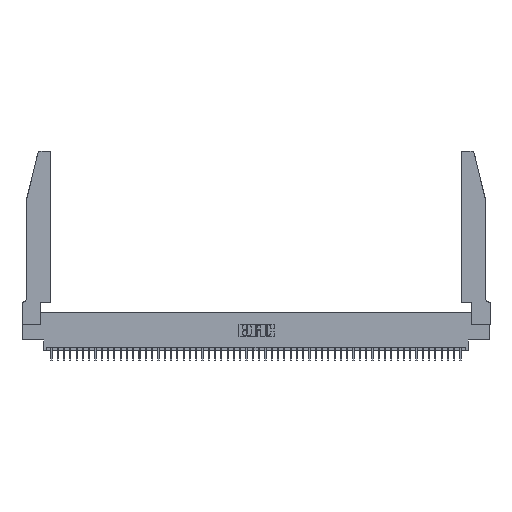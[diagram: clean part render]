
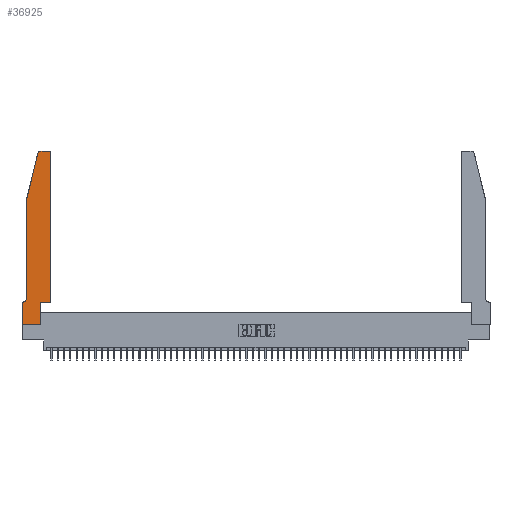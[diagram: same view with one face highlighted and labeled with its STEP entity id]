
A CAD part, top view. The second image highlights one B-rep face of the part: STEP entity #36925.
In plain terms, the highlighted planar face has unit normal (0, 0, 1).
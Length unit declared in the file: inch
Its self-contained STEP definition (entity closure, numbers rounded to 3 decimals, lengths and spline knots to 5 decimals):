
#589 = DIRECTION ( 'NONE',  ( -1., 0., 0. ) ) ;
#664 = CARTESIAN_POINT ( 'NONE',  ( 0.4505, 2.72, 0.37 ) ) ;
#1329 = VERTEX_POINT ( 'NONE', #664 ) ;
#1554 = VERTEX_POINT ( 'NONE', #31294 ) ;
#1745 = EDGE_CURVE ( 'NONE', #17024, #6309, #14048, .T. ) ;
#1891 = EDGE_CURVE ( 'NONE', #22762, #1329, #19160, .T. ) ;
#2009 = ORIENTED_EDGE ( 'NONE', *, *, #38502, .T. ) ;
#2164 = EDGE_CURVE ( 'NONE', #41203, #17024, #21786, .T. ) ;
#2355 = VERTEX_POINT ( 'NONE', #8171 ) ;
#2985 = CARTESIAN_POINT ( 'NONE',  ( 0., 0.35, 0.37 ) ) ;
#3336 = VERTEX_POINT ( 'NONE', #47160 ) ;
#3424 = EDGE_CURVE ( 'NONE', #1329, #51830, #41658, .T. ) ;
#3543 = VECTOR ( 'NONE', #29038, 39.37008 ) ;
#3907 = DIRECTION ( 'NONE',  ( 0., 0., 1. ) ) ;
#4087 = DIRECTION ( 'NONE',  ( 0., 1., 0. ) ) ;
#4681 = ORIENTED_EDGE ( 'NONE', *, *, #37167, .T. ) ;
#5021 = DIRECTION ( 'NONE',  ( 0., 0., -1. ) ) ;
#5131 = ORIENTED_EDGE ( 'NONE', *, *, #1891, .T. ) ;
#6309 = VERTEX_POINT ( 'NONE', #47322 ) ;
#6726 = DIRECTION ( 'NONE',  ( 1., 0., 0. ) ) ;
#6755 = FACE_OUTER_BOUND ( 'NONE', #8197, .T. ) ;
#8171 = CARTESIAN_POINT ( 'NONE',  ( 0.0055, 0.35, 0.37 ) ) ;
#8197 = EDGE_LOOP ( 'NONE', ( #2009, #19649, #50811, #50943, #4681, #10469, #21205, #13644, #23918, #22284, #5131, #49922 ) ) ;
#9561 = EDGE_CURVE ( 'NONE', #21285, #1554, #14188, .T. ) ;
#10469 = ORIENTED_EDGE ( 'NONE', *, *, #12463, .T. ) ;
#10592 = DIRECTION ( 'NONE',  ( -0.239, -0.971, 0. ) ) ;
#12463 = EDGE_CURVE ( 'NONE', #2355, #21559, #24625, .T. ) ;
#12718 = VECTOR ( 'NONE', #13935, 39.37008 ) ;
#12909 = VECTOR ( 'NONE', #47338, 39.37008 ) ;
#13644 = ORIENTED_EDGE ( 'NONE', *, *, #41360, .T. ) ;
#13935 = DIRECTION ( 'NONE',  ( 0., -1., 0. ) ) ;
#14048 = LINE ( 'NONE', #34669, #45701 ) ;
#14188 = LINE ( 'NONE', #51188, #12909 ) ;
#15741 = CARTESIAN_POINT ( 'NONE',  ( 0.284, 2.75, 0.37 ) ) ;
#16290 = VERTEX_POINT ( 'NONE', #39798 ) ;
#16365 = DIRECTION ( 'NONE',  ( 1., 0., 0. ) ) ;
#17024 = VERTEX_POINT ( 'NONE', #51663 ) ;
#17715 = AXIS2_PLACEMENT_3D ( 'NONE', #23643, #48736, #36466 ) ;
#17848 = LINE ( 'NONE', #18419, #12718 ) ;
#18419 = CARTESIAN_POINT ( 'NONE',  ( 0.0755, 2., 0.37 ) ) ;
#18523 = DIRECTION ( 'NONE',  ( -1., 0., 0. ) ) ;
#18718 = DIRECTION ( 'NONE',  ( 1., 0., 0. ) ) ;
#19160 = LINE ( 'NONE', #45069, #31456 ) ;
#19649 = ORIENTED_EDGE ( 'NONE', *, *, #2164, .T. ) ;
#19700 = LINE ( 'NONE', #43746, #44237 ) ;
#21143 = CARTESIAN_POINT ( 'NONE',  ( 0.2865, 0., 0.37 ) ) ;
#21205 = ORIENTED_EDGE ( 'NONE', *, *, #47074, .T. ) ;
#21285 = VERTEX_POINT ( 'NONE', #21143 ) ;
#21559 = VERTEX_POINT ( 'NONE', #2985 ) ;
#21786 = CIRCLE ( 'NONE', #44811, 0.03 ) ;
#22284 = ORIENTED_EDGE ( 'NONE', *, *, #43939, .T. ) ;
#22672 = CARTESIAN_POINT ( 'NONE',  ( 0.0755, 0.35, 0.37 ) ) ;
#22712 = DIRECTION ( 'NONE',  ( 0., 0., 1. ) ) ;
#22762 = VERTEX_POINT ( 'NONE', #39744 ) ;
#23643 = CARTESIAN_POINT ( 'NONE',  ( 0., 0.35, 0.37 ) ) ;
#23918 = ORIENTED_EDGE ( 'NONE', *, *, #9561, .T. ) ;
#24625 = LINE ( 'NONE', #22672, #53123 ) ;
#25334 = CARTESIAN_POINT ( 'NONE',  ( 0.2605, 2.75, 0.37 ) ) ;
#27269 = VECTOR ( 'NONE', #589, 39.37008 ) ;
#27947 = CARTESIAN_POINT ( 'NONE',  ( 0.284, 2.72, 0.37 ) ) ;
#29038 = DIRECTION ( 'NONE',  ( 0., -1., 0. ) ) ;
#31294 = CARTESIAN_POINT ( 'NONE',  ( 0.2865, 0.35, 0.37 ) ) ;
#31456 = VECTOR ( 'NONE', #4087, 39.37008 ) ;
#32135 = PLANE ( 'NONE',  #17715 ) ;
#34481 = CARTESIAN_POINT ( 'NONE',  ( 0., 0., 0.37 ) ) ;
#34669 = CARTESIAN_POINT ( 'NONE',  ( 0.0755, 2., 0.37 ) ) ;
#35971 = LINE ( 'NONE', #34481, #53486 ) ;
#36466 = DIRECTION ( 'NONE',  ( 1., 0., 0. ) ) ;
#36925 = ADVANCED_FACE ( 'NONE', ( #6755 ), #32135, .T. ) ;
#37167 = EDGE_CURVE ( 'NONE', #16290, #2355, #51346, .T. ) ;
#38269 = CARTESIAN_POINT ( 'NONE',  ( 0.0055, 0.42, 0.37 ) ) ;
#38502 = EDGE_CURVE ( 'NONE', #51830, #41203, #42133, .T. ) ;
#39486 = CARTESIAN_POINT ( 'NONE',  ( 0.4205, 2.72, 0.37 ) ) ;
#39744 = CARTESIAN_POINT ( 'NONE',  ( 0.4505, 0.35, 0.37 ) ) ;
#39798 = CARTESIAN_POINT ( 'NONE',  ( 0.0755, 0.42, 0.37 ) ) ;
#40934 = CARTESIAN_POINT ( 'NONE',  ( 0., 0., 0.37 ) ) ;
#41203 = VERTEX_POINT ( 'NONE', #15741 ) ;
#41360 = EDGE_CURVE ( 'NONE', #3336, #21285, #35971, .T. ) ;
#41658 = CIRCLE ( 'NONE', #51118, 0.03 ) ;
#42133 = LINE ( 'NONE', #25334, #27269 ) ;
#43746 = CARTESIAN_POINT ( 'NONE',  ( 0.4505, 0.35, 0.37 ) ) ;
#43939 = EDGE_CURVE ( 'NONE', #1554, #22762, #19700, .T. ) ;
#44237 = VECTOR ( 'NONE', #6726, 39.37008 ) ;
#44811 = AXIS2_PLACEMENT_3D ( 'NONE', #27947, #3907, #16365 ) ;
#45069 = CARTESIAN_POINT ( 'NONE',  ( 0.4505, 0.35, 0.37 ) ) ;
#45701 = VECTOR ( 'NONE', #10592, 39.37008 ) ;
#46585 = EDGE_CURVE ( 'NONE', #6309, #16290, #17848, .T. ) ;
#46888 = LINE ( 'NONE', #40934, #3543 ) ;
#47074 = EDGE_CURVE ( 'NONE', #21559, #3336, #46888, .T. ) ;
#47160 = CARTESIAN_POINT ( 'NONE',  ( 0., 0., 0.37 ) ) ;
#47322 = CARTESIAN_POINT ( 'NONE',  ( 0.0755, 2., 0.37 ) ) ;
#47338 = DIRECTION ( 'NONE',  ( 0., 1., 0. ) ) ;
#47619 = DIRECTION ( 'NONE',  ( 1., 0., 0. ) ) ;
#48135 = AXIS2_PLACEMENT_3D ( 'NONE', #38269, #5021, #49823 ) ;
#48736 = DIRECTION ( 'NONE',  ( 0., 0., 1. ) ) ;
#49071 = CARTESIAN_POINT ( 'NONE',  ( 0.4205, 2.75, 0.37 ) ) ;
#49823 = DIRECTION ( 'NONE',  ( -1., 0., 0. ) ) ;
#49922 = ORIENTED_EDGE ( 'NONE', *, *, #3424, .T. ) ;
#50811 = ORIENTED_EDGE ( 'NONE', *, *, #1745, .T. ) ;
#50943 = ORIENTED_EDGE ( 'NONE', *, *, #46585, .T. ) ;
#51118 = AXIS2_PLACEMENT_3D ( 'NONE', #39486, #22712, #47619 ) ;
#51188 = CARTESIAN_POINT ( 'NONE',  ( 0.2865, 0.35, 0.37 ) ) ;
#51346 = CIRCLE ( 'NONE', #48135, 0.07 ) ;
#51663 = CARTESIAN_POINT ( 'NONE',  ( 0.25487, 2.72718, 0.37 ) ) ;
#51830 = VERTEX_POINT ( 'NONE', #49071 ) ;
#53123 = VECTOR ( 'NONE', #18523, 39.37008 ) ;
#53486 = VECTOR ( 'NONE', #18718, 39.37008 ) ;
